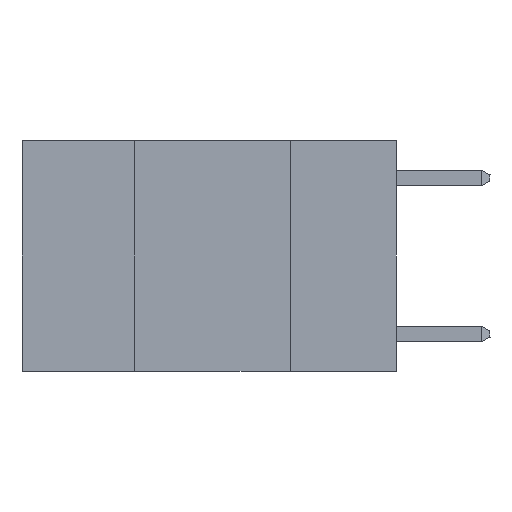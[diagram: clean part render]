
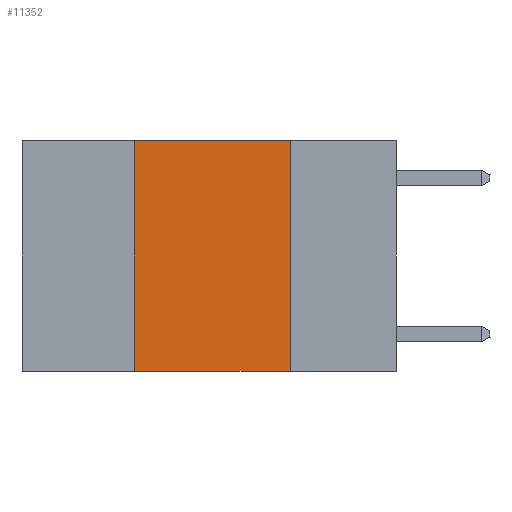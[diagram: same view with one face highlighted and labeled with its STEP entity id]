
A CAD part, left-side view. The second image highlights one B-rep face of the part: STEP entity #11352.
In plain terms, the highlighted planar face has unit normal (-1, 0, 0).
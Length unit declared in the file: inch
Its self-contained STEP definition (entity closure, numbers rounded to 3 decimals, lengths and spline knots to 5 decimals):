
#78 = CARTESIAN_POINT ( 'NONE',  ( 0., 0.42, 0. ) ) ;
#537 = DIRECTION ( 'NONE',  ( 0., 0., 1. ) ) ;
#626 = FACE_OUTER_BOUND ( 'NONE', #3479, .T. ) ;
#820 = VECTOR ( 'NONE', #3250, 39.37008 ) ;
#997 = CARTESIAN_POINT ( 'NONE',  ( 0., 0.6, -0.37 ) ) ;
#1035 = CARTESIAN_POINT ( 'NONE',  ( 0., 0.17, -0.37 ) ) ;
#1682 = LINE ( 'NONE', #9834, #6148 ) ;
#1991 = ORIENTED_EDGE ( 'NONE', *, *, #3527, .F. ) ;
#2891 = DIRECTION ( 'NONE',  ( 0., -1., 0. ) ) ;
#3104 = VECTOR ( 'NONE', #537, 39.37008 ) ;
#3250 = DIRECTION ( 'NONE',  ( 0., -1., 0. ) ) ;
#3479 = EDGE_LOOP ( 'NONE', ( #1991, #4984, #8580, #7606 ) ) ;
#3527 = EDGE_CURVE ( 'NONE', #8228, #7979, #1682, .T. ) ;
#3681 = VERTEX_POINT ( 'NONE', #10130 ) ;
#4780 = VERTEX_POINT ( 'NONE', #78 ) ;
#4984 = ORIENTED_EDGE ( 'NONE', *, *, #9632, .F. ) ;
#5127 = LINE ( 'NONE', #6028, #820 ) ;
#5230 = CARTESIAN_POINT ( 'NONE',  ( 0., 0.6, 0. ) ) ;
#6028 = CARTESIAN_POINT ( 'NONE',  ( 0., 0.6, 0. ) ) ;
#6148 = VECTOR ( 'NONE', #8074, 39.37008 ) ;
#6636 = AXIS2_PLACEMENT_3D ( 'NONE', #5230, #11680, #9519 ) ;
#7339 = EDGE_CURVE ( 'NONE', #3681, #4780, #8797, .T. ) ;
#7371 = VECTOR ( 'NONE', #2891, 39.37008 ) ;
#7606 = ORIENTED_EDGE ( 'NONE', *, *, #9548, .T. ) ;
#7979 = VERTEX_POINT ( 'NONE', #1035 ) ;
#8074 = DIRECTION ( 'NONE',  ( 0., 0., -1. ) ) ;
#8228 = VERTEX_POINT ( 'NONE', #11483 ) ;
#8534 = PLANE ( 'NONE',  #6636 ) ;
#8580 = ORIENTED_EDGE ( 'NONE', *, *, #7339, .F. ) ;
#8613 = CARTESIAN_POINT ( 'NONE',  ( 0., 0.42, 0. ) ) ;
#8797 = LINE ( 'NONE', #8613, #3104 ) ;
#9519 = DIRECTION ( 'NONE',  ( 0., 0., -1. ) ) ;
#9548 = EDGE_CURVE ( 'NONE', #3681, #7979, #10421, .T. ) ;
#9632 = EDGE_CURVE ( 'NONE', #4780, #8228, #5127, .T. ) ;
#9834 = CARTESIAN_POINT ( 'NONE',  ( 0., 0.17, 0. ) ) ;
#10130 = CARTESIAN_POINT ( 'NONE',  ( 0., 0.42, -0.37 ) ) ;
#10421 = LINE ( 'NONE', #997, #7371 ) ;
#11352 = ADVANCED_FACE ( 'NONE', ( #626 ), #8534, .F. ) ;
#11483 = CARTESIAN_POINT ( 'NONE',  ( 0., 0.17, 0. ) ) ;
#11680 = DIRECTION ( 'NONE',  ( 1., 0., 0. ) ) ;
